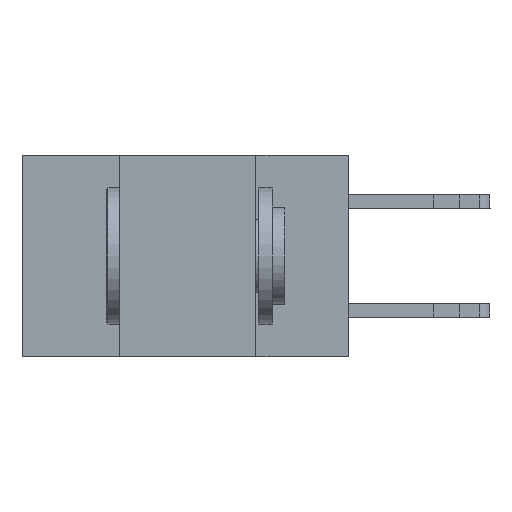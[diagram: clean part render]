
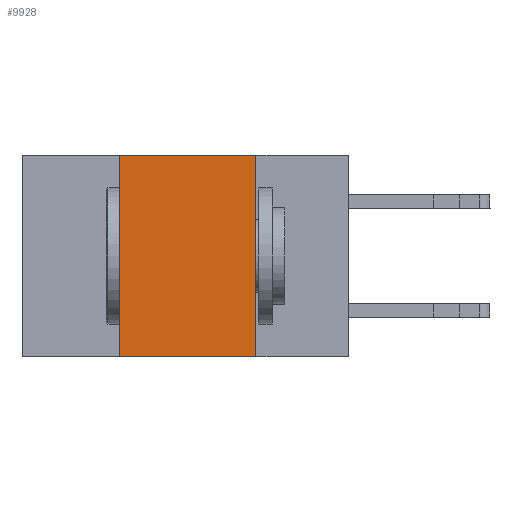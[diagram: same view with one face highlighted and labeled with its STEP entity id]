
A CAD part, left-side view. The second image highlights one B-rep face of the part: STEP entity #9928.
In plain terms, the highlighted planar face has unit normal (-1, 0, 0).
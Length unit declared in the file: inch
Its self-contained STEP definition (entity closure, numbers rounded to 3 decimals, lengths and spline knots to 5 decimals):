
#178 = VERTEX_POINT ( 'NONE', #17515 ) ;
#988 = ORIENTED_EDGE ( 'NONE', *, *, #5493, .F. ) ;
#1386 = AXIS2_PLACEMENT_3D ( 'NONE', #18029, #9220, #3577 ) ;
#1605 = DIRECTION ( 'NONE',  ( 0., -1., 0. ) ) ;
#2367 = VECTOR ( 'NONE', #2977, 39.37008 ) ;
#2374 = EDGE_LOOP ( 'NONE', ( #8161, #6622, #988, #4181 ) ) ;
#2439 = VECTOR ( 'NONE', #12355, 39.37008 ) ;
#2977 = DIRECTION ( 'NONE',  ( 0., -1., 0. ) ) ;
#2981 = EDGE_CURVE ( 'NONE', #6801, #17419, #17236, .T. ) ;
#3420 = CARTESIAN_POINT ( 'NONE',  ( 0., 0.42, -0.37 ) ) ;
#3481 = PLANE ( 'NONE',  #1386 ) ;
#3544 = CARTESIAN_POINT ( 'NONE',  ( 0., 0.6, 0. ) ) ;
#3577 = DIRECTION ( 'NONE',  ( 0., 0., -1. ) ) ;
#3873 = DIRECTION ( 'NONE',  ( 0., 0., -1. ) ) ;
#3996 = LINE ( 'NONE', #17968, #2439 ) ;
#4181 = ORIENTED_EDGE ( 'NONE', *, *, #2981, .T. ) ;
#4455 = VECTOR ( 'NONE', #3873, 39.37008 ) ;
#5493 = EDGE_CURVE ( 'NONE', #6801, #9294, #3996, .T. ) ;
#6110 = VECTOR ( 'NONE', #1605, 39.37008 ) ;
#6622 = ORIENTED_EDGE ( 'NONE', *, *, #8278, .F. ) ;
#6801 = VERTEX_POINT ( 'NONE', #3420 ) ;
#6894 = CARTESIAN_POINT ( 'NONE',  ( 0., 0.17, -0.37 ) ) ;
#8161 = ORIENTED_EDGE ( 'NONE', *, *, #12363, .F. ) ;
#8278 = EDGE_CURVE ( 'NONE', #9294, #178, #16401, .T. ) ;
#9220 = DIRECTION ( 'NONE',  ( 1., 0., 0. ) ) ;
#9294 = VERTEX_POINT ( 'NONE', #14337 ) ;
#9928 = ADVANCED_FACE ( 'NONE', ( #12229 ), #3481, .F. ) ;
#12229 = FACE_OUTER_BOUND ( 'NONE', #2374, .T. ) ;
#12355 = DIRECTION ( 'NONE',  ( 0., 0., 1. ) ) ;
#12363 = EDGE_CURVE ( 'NONE', #178, #17419, #13833, .T. ) ;
#13833 = LINE ( 'NONE', #6894, #4455 ) ;
#14337 = CARTESIAN_POINT ( 'NONE',  ( 0., 0.42, 0. ) ) ;
#15836 = CARTESIAN_POINT ( 'NONE',  ( 0., 0.6, -0.37 ) ) ;
#16401 = LINE ( 'NONE', #3544, #6110 ) ;
#17236 = LINE ( 'NONE', #15836, #2367 ) ;
#17313 = CARTESIAN_POINT ( 'NONE',  ( 0., 0.17, -0.37 ) ) ;
#17419 = VERTEX_POINT ( 'NONE', #17313 ) ;
#17515 = CARTESIAN_POINT ( 'NONE',  ( 0., 0.17, 0. ) ) ;
#17968 = CARTESIAN_POINT ( 'NONE',  ( 0., 0.42, -0.37 ) ) ;
#18029 = CARTESIAN_POINT ( 'NONE',  ( 0., 0.6, 0. ) ) ;
